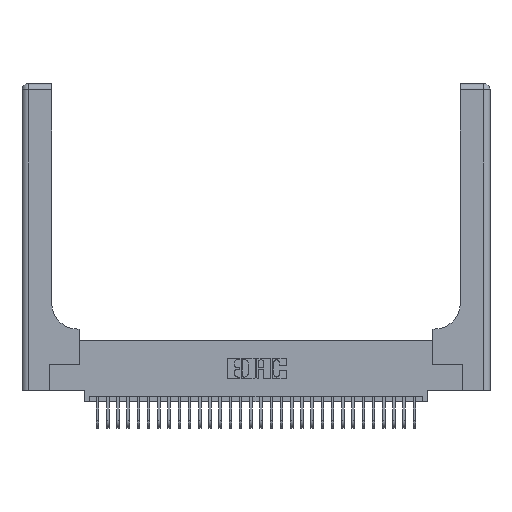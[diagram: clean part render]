
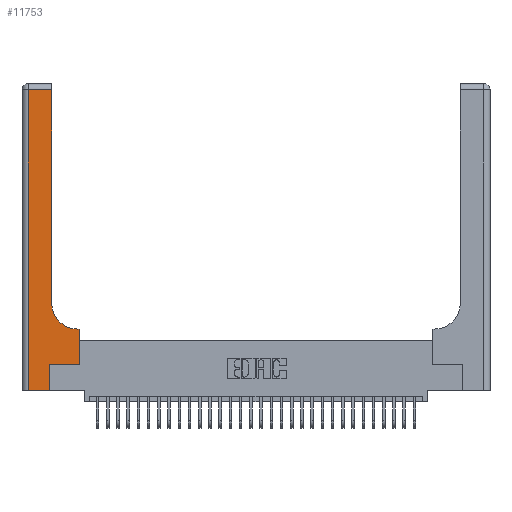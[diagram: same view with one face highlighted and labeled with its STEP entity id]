
A CAD part, top view. The second image highlights one B-rep face of the part: STEP entity #11753.
In plain terms, the highlighted planar face has unit normal (0, 0, 1).
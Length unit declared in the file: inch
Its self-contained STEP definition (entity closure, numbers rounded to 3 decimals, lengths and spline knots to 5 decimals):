
#2227 = VECTOR ( 'NONE', #25587, 39.37008 ) ;
#2464 = CARTESIAN_POINT ( 'NONE',  ( 0.5585, 0.6, 0.37 ) ) ;
#2503 = DIRECTION ( 'NONE',  ( 0., 1., 0. ) ) ;
#2766 = FACE_OUTER_BOUND ( 'NONE', #9601, .T. ) ;
#3236 = VERTEX_POINT ( 'NONE', #25498 ) ;
#3569 = PLANE ( 'NONE',  #15161 ) ;
#3659 = VERTEX_POINT ( 'NONE', #22777 ) ;
#3765 = AXIS2_PLACEMENT_3D ( 'NONE', #11664, #28266, #14072 ) ;
#4063 = VECTOR ( 'NONE', #16871, 39.37008 ) ;
#4517 = CARTESIAN_POINT ( 'NONE',  ( 0.2915, 0.85, 0.37 ) ) ;
#4851 = EDGE_CURVE ( 'NONE', #24338, #16235, #16794, .T. ) ;
#4992 = CARTESIAN_POINT ( 'NONE',  ( 0.2915, 3., 0.37 ) ) ;
#6209 = ORIENTED_EDGE ( 'NONE', *, *, #23601, .T. ) ;
#8050 = VECTOR ( 'NONE', #12882, 39.37008 ) ;
#8370 = CARTESIAN_POINT ( 'NONE',  ( 0.2915, 0.6, 0.37 ) ) ;
#8522 = DIRECTION ( 'NONE',  ( 1., 0., 0. ) ) ;
#9601 = EDGE_LOOP ( 'NONE', ( #13454, #6209, #27728, #17776, #20803, #13434, #17137, #26078, #19244 ) ) ;
#10762 = CARTESIAN_POINT ( 'NONE',  ( 0., 3., 0.37 ) ) ;
#11139 = CARTESIAN_POINT ( 'NONE',  ( 0.5585, 0.25, 0.37 ) ) ;
#11613 = LINE ( 'NONE', #16788, #18710 ) ;
#11630 = LINE ( 'NONE', #20408, #22792 ) ;
#11664 = CARTESIAN_POINT ( 'NONE',  ( 0.5415, 0.85, 0.37 ) ) ;
#11753 = ADVANCED_FACE ( 'NONE', ( #2766 ), #3569, .F. ) ;
#12532 = EDGE_CURVE ( 'NONE', #16235, #19586, #22180, .T. ) ;
#12882 = DIRECTION ( 'NONE',  ( 1., 0., 0. ) ) ;
#13149 = DIRECTION ( 'NONE',  ( -1., 0., 0. ) ) ;
#13434 = ORIENTED_EDGE ( 'NONE', *, *, #28062, .T. ) ;
#13454 = ORIENTED_EDGE ( 'NONE', *, *, #23759, .T. ) ;
#13610 = VERTEX_POINT ( 'NONE', #13791 ) ;
#13753 = LINE ( 'NONE', #11139, #19341 ) ;
#13791 = CARTESIAN_POINT ( 'NONE',  ( 0.2915, 2.94, 0.37 ) ) ;
#14072 = DIRECTION ( 'NONE',  ( 1., 0., 0. ) ) ;
#14181 = DIRECTION ( 'NONE',  ( 0., -1., 0. ) ) ;
#15161 = AXIS2_PLACEMENT_3D ( 'NONE', #10762, #27372, #13149 ) ;
#15891 = LINE ( 'NONE', #29487, #8050 ) ;
#16235 = VERTEX_POINT ( 'NONE', #30143 ) ;
#16788 = CARTESIAN_POINT ( 'NONE',  ( 0.269, 0., 0.37 ) ) ;
#16794 = LINE ( 'NONE', #8370, #17530 ) ;
#16871 = DIRECTION ( 'NONE',  ( 0., 1., 0. ) ) ;
#16934 = VERTEX_POINT ( 'NONE', #30417 ) ;
#17137 = ORIENTED_EDGE ( 'NONE', *, *, #29773, .T. ) ;
#17530 = VECTOR ( 'NONE', #25005, 39.37008 ) ;
#17776 = ORIENTED_EDGE ( 'NONE', *, *, #26115, .T. ) ;
#18710 = VECTOR ( 'NONE', #2503, 39.37008 ) ;
#19244 = ORIENTED_EDGE ( 'NONE', *, *, #12532, .T. ) ;
#19341 = VECTOR ( 'NONE', #27758, 39.37008 ) ;
#19586 = VERTEX_POINT ( 'NONE', #4517 ) ;
#19750 = LINE ( 'NONE', #28372, #26780 ) ;
#20408 = CARTESIAN_POINT ( 'NONE',  ( 0.269, 0.25, 0.37 ) ) ;
#20803 = ORIENTED_EDGE ( 'NONE', *, *, #22584, .T. ) ;
#21257 = LINE ( 'NONE', #23221, #2227 ) ;
#22180 = CIRCLE ( 'NONE', #3765, 0.25 ) ;
#22584 = EDGE_CURVE ( 'NONE', #3236, #16934, #11613, .T. ) ;
#22777 = CARTESIAN_POINT ( 'NONE',  ( 0.06, 0., 0.37 ) ) ;
#22792 = VECTOR ( 'NONE', #8522, 39.37008 ) ;
#23181 = VERTEX_POINT ( 'NONE', #23497 ) ;
#23221 = CARTESIAN_POINT ( 'NONE',  ( 0., 2.94, 0.37 ) ) ;
#23497 = CARTESIAN_POINT ( 'NONE',  ( 0.06, 2.94, 0.37 ) ) ;
#23601 = EDGE_CURVE ( 'NONE', #13610, #23181, #21257, .T. ) ;
#23649 = EDGE_CURVE ( 'NONE', #23181, #3659, #19750, .T. ) ;
#23759 = EDGE_CURVE ( 'NONE', #19586, #13610, #28606, .T. ) ;
#24338 = VERTEX_POINT ( 'NONE', #2464 ) ;
#25005 = DIRECTION ( 'NONE',  ( -1., 0., 0. ) ) ;
#25288 = VERTEX_POINT ( 'NONE', #25801 ) ;
#25498 = CARTESIAN_POINT ( 'NONE',  ( 0.269, 0., 0.37 ) ) ;
#25587 = DIRECTION ( 'NONE',  ( -1., 0., 0. ) ) ;
#25801 = CARTESIAN_POINT ( 'NONE',  ( 0.5585, 0.25, 0.37 ) ) ;
#26078 = ORIENTED_EDGE ( 'NONE', *, *, #4851, .T. ) ;
#26115 = EDGE_CURVE ( 'NONE', #3659, #3236, #15891, .T. ) ;
#26780 = VECTOR ( 'NONE', #14181, 39.37008 ) ;
#27372 = DIRECTION ( 'NONE',  ( 0., 0., -1. ) ) ;
#27728 = ORIENTED_EDGE ( 'NONE', *, *, #23649, .T. ) ;
#27758 = DIRECTION ( 'NONE',  ( 0., 1., 0. ) ) ;
#28062 = EDGE_CURVE ( 'NONE', #16934, #25288, #11630, .T. ) ;
#28266 = DIRECTION ( 'NONE',  ( 0., 0., -1. ) ) ;
#28372 = CARTESIAN_POINT ( 'NONE',  ( 0.06, 3., 0.37 ) ) ;
#28606 = LINE ( 'NONE', #4992, #4063 ) ;
#29487 = CARTESIAN_POINT ( 'NONE',  ( 0., 0., 0.37 ) ) ;
#29773 = EDGE_CURVE ( 'NONE', #25288, #24338, #13753, .T. ) ;
#30143 = CARTESIAN_POINT ( 'NONE',  ( 0.5415, 0.6, 0.37 ) ) ;
#30417 = CARTESIAN_POINT ( 'NONE',  ( 0.269, 0.25, 0.37 ) ) ;
